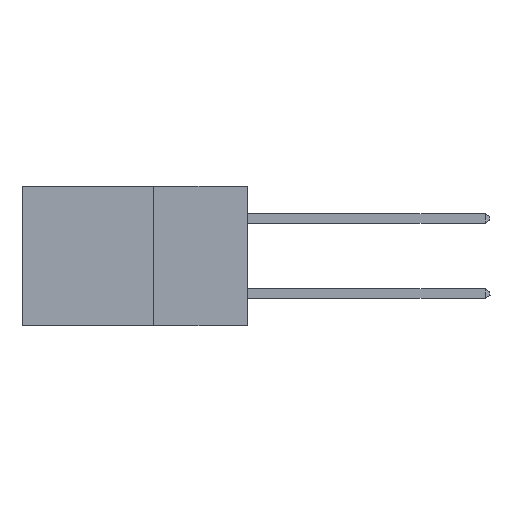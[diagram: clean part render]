
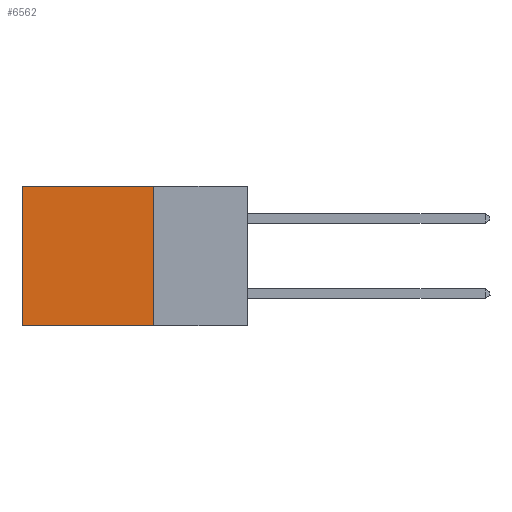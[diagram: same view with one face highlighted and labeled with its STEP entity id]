
A CAD part, left-side view. The second image highlights one B-rep face of the part: STEP entity #6562.
In plain terms, the highlighted planar face has unit normal (-1, 0, 0).
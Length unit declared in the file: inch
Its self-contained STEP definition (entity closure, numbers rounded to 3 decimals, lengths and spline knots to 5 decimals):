
#155 = DIRECTION ( 'NONE',  ( 0., 0., -1. ) ) ;
#1332 = VERTEX_POINT ( 'NONE', #2666 ) ;
#1857 = CARTESIAN_POINT ( 'NONE',  ( 0.298, 0.6, 0. ) ) ;
#2094 = LINE ( 'NONE', #25743, #13166 ) ;
#2666 = CARTESIAN_POINT ( 'NONE',  ( 0.298, 0.25, -0.37 ) ) ;
#2716 = DIRECTION ( 'NONE',  ( 0., 1., 0. ) ) ;
#3554 = VECTOR ( 'NONE', #10312, 39.37008 ) ;
#3707 = VERTEX_POINT ( 'NONE', #23397 ) ;
#3792 = DIRECTION ( 'NONE',  ( 0., 0., -1. ) ) ;
#5421 = VERTEX_POINT ( 'NONE', #22894 ) ;
#5893 = ORIENTED_EDGE ( 'NONE', *, *, #10020, .T. ) ;
#6196 = FACE_OUTER_BOUND ( 'NONE', #7116, .T. ) ;
#6562 = ADVANCED_FACE ( 'NONE', ( #6196 ), #16151, .F. ) ;
#7116 = EDGE_LOOP ( 'NONE', ( #7741, #15678, #9194, #5893 ) ) ;
#7409 = VERTEX_POINT ( 'NONE', #8972 ) ;
#7741 = ORIENTED_EDGE ( 'NONE', *, *, #24144, .T. ) ;
#8044 = CARTESIAN_POINT ( 'NONE',  ( 0.298, 0.25, 0. ) ) ;
#8221 = AXIS2_PLACEMENT_3D ( 'NONE', #8044, #22166, #155 ) ;
#8972 = CARTESIAN_POINT ( 'NONE',  ( 0.298, 0.6, 0. ) ) ;
#9194 = ORIENTED_EDGE ( 'NONE', *, *, #24069, .F. ) ;
#9885 = CARTESIAN_POINT ( 'NONE',  ( 0.298, 0.25, 0. ) ) ;
#10020 = EDGE_CURVE ( 'NONE', #3707, #7409, #2094, .T. ) ;
#10312 = DIRECTION ( 'NONE',  ( 0., 0., -1. ) ) ;
#13166 = VECTOR ( 'NONE', #13686, 39.37008 ) ;
#13686 = DIRECTION ( 'NONE',  ( 0., 1., 0. ) ) ;
#14531 = VECTOR ( 'NONE', #2716, 39.37008 ) ;
#15678 = ORIENTED_EDGE ( 'NONE', *, *, #24523, .F. ) ;
#15863 = LINE ( 'NONE', #1857, #3554 ) ;
#16151 = PLANE ( 'NONE',  #8221 ) ;
#19603 = VECTOR ( 'NONE', #3792, 39.37008 ) ;
#21151 = CARTESIAN_POINT ( 'NONE',  ( 0.298, 0.25, -0.37 ) ) ;
#22166 = DIRECTION ( 'NONE',  ( 1., 0., 0. ) ) ;
#22894 = CARTESIAN_POINT ( 'NONE',  ( 0.298, 0.6, -0.37 ) ) ;
#23397 = CARTESIAN_POINT ( 'NONE',  ( 0.298, 0.25, 0. ) ) ;
#24069 = EDGE_CURVE ( 'NONE', #3707, #1332, #25314, .T. ) ;
#24144 = EDGE_CURVE ( 'NONE', #7409, #5421, #15863, .T. ) ;
#24523 = EDGE_CURVE ( 'NONE', #1332, #5421, #24991, .T. ) ;
#24991 = LINE ( 'NONE', #21151, #14531 ) ;
#25314 = LINE ( 'NONE', #9885, #19603 ) ;
#25743 = CARTESIAN_POINT ( 'NONE',  ( 0.298, 0.25, 0. ) ) ;
